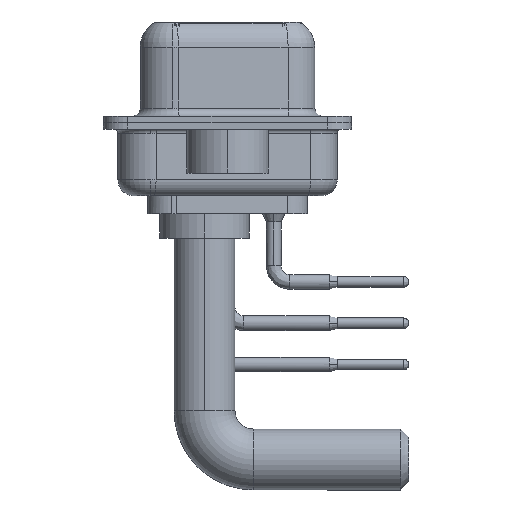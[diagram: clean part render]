
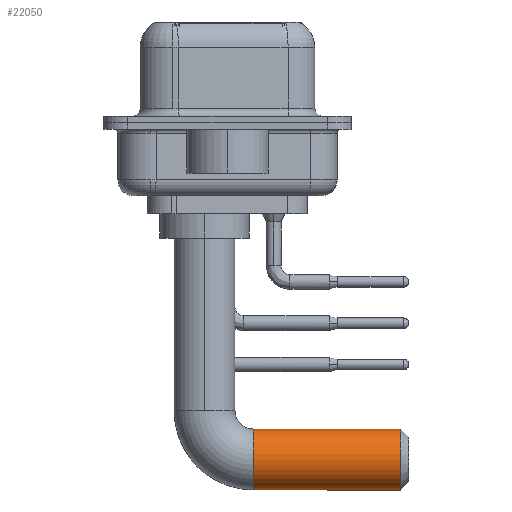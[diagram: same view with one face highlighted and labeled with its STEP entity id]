
A CAD part, left-side view. The second image highlights one B-rep face of the part: STEP entity #22050.
In plain terms, the highlighted cylindrical face has radius 1.875 mm (diameter 3.75 mm), a partial arc.
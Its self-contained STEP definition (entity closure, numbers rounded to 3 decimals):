
#84 = DIRECTION ( 'NONE',  ( 0., -1., 0. ) ) ;
#351 = VECTOR ( 'NONE', #19345, 1000. ) ;
#2321 = CYLINDRICAL_SURFACE ( 'NONE', #19001, 1.875 ) ;
#3563 = LINE ( 'NONE', #5970, #351 ) ;
#4815 = VERTEX_POINT ( 'NONE', #14787 ) ;
#4912 = DIRECTION ( 'NONE',  ( 0., 0., -1. ) ) ;
#5212 = CARTESIAN_POINT ( 'NONE',  ( 0., -3., -13.63 ) ) ;
#5263 = ORIENTED_EDGE ( 'NONE', *, *, #5633, .T. ) ;
#5633 = EDGE_CURVE ( 'NONE', #16743, #11879, #23382, .T. ) ;
#5970 = CARTESIAN_POINT ( 'NONE',  ( 0., -3., -15.505 ) ) ;
#5997 = ORIENTED_EDGE ( 'NONE', *, *, #33764, .T. ) ;
#6310 = DIRECTION ( 'NONE',  ( 0., -1., 0. ) ) ;
#7306 = DIRECTION ( 'NONE',  ( -1., 0., 0. ) ) ;
#8531 = ORIENTED_EDGE ( 'NONE', *, *, #21386, .T. ) ;
#10197 = FACE_OUTER_BOUND ( 'NONE', #25750, .T. ) ;
#10231 = CARTESIAN_POINT ( 'NONE',  ( 0., -12.07, -13.63 ) ) ;
#10310 = ORIENTED_EDGE ( 'NONE', *, *, #13794, .F. ) ;
#11879 = VERTEX_POINT ( 'NONE', #24050 ) ;
#12064 = CARTESIAN_POINT ( 'NONE',  ( 0., -12.07, -15.505 ) ) ;
#12628 = DIRECTION ( 'NONE',  ( 0., 1., 0. ) ) ;
#13794 = EDGE_CURVE ( 'NONE', #4815, #11879, #29678, .T. ) ;
#13863 = CARTESIAN_POINT ( 'NONE',  ( 0., -3., -11.755 ) ) ;
#14787 = CARTESIAN_POINT ( 'NONE',  ( 0., -3., -11.755 ) ) ;
#16743 = VERTEX_POINT ( 'NONE', #12064 ) ;
#17247 = CARTESIAN_POINT ( 'NONE',  ( 0., -3., -13.63 ) ) ;
#19001 = AXIS2_PLACEMENT_3D ( 'NONE', #5212, #84, #33895 ) ;
#19345 = DIRECTION ( 'NONE',  ( 0., -1., 0. ) ) ;
#21386 = EDGE_CURVE ( 'NONE', #30208, #16743, #3563, .T. ) ;
#22050 = ADVANCED_FACE ( 'NONE', ( #10197 ), #2321, .T. ) ;
#22946 = DIRECTION ( 'NONE',  ( 0., -1., 0. ) ) ;
#23382 = CIRCLE ( 'NONE', #29406, 1.875 ) ;
#24050 = CARTESIAN_POINT ( 'NONE',  ( 0., -12.07, -11.755 ) ) ;
#25750 = EDGE_LOOP ( 'NONE', ( #10310, #5997, #8531, #5263 ) ) ;
#29406 = AXIS2_PLACEMENT_3D ( 'NONE', #10231, #12628, #4912 ) ;
#29536 = CARTESIAN_POINT ( 'NONE',  ( 0., -3., -15.505 ) ) ;
#29678 = LINE ( 'NONE', #13863, #29769 ) ;
#29769 = VECTOR ( 'NONE', #6310, 1000. ) ;
#30208 = VERTEX_POINT ( 'NONE', #29536 ) ;
#30322 = AXIS2_PLACEMENT_3D ( 'NONE', #17247, #22946, #7306 ) ;
#33060 = CIRCLE ( 'NONE', #30322, 1.875 ) ;
#33764 = EDGE_CURVE ( 'NONE', #4815, #30208, #33060, .T. ) ;
#33895 = DIRECTION ( 'NONE',  ( 0., 0., -1. ) ) ;
